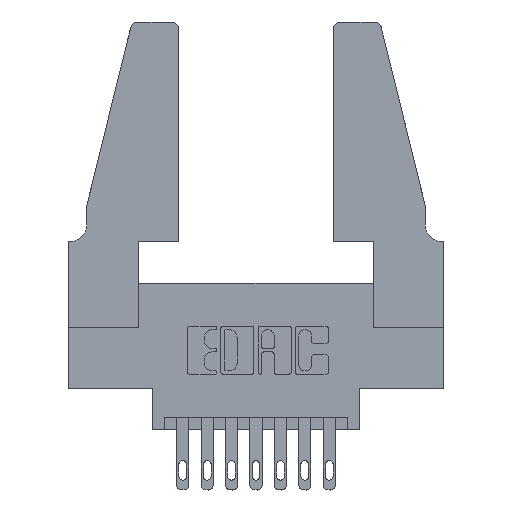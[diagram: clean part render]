
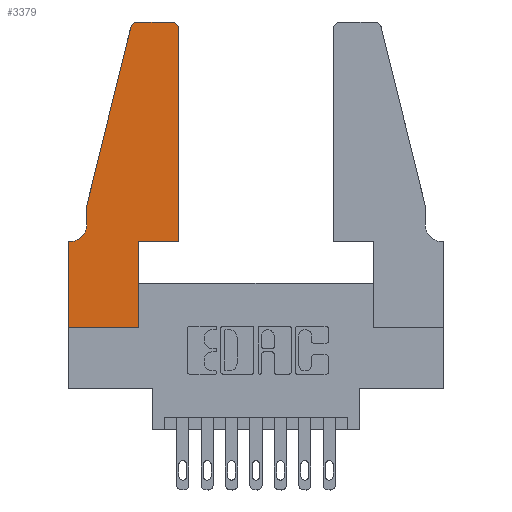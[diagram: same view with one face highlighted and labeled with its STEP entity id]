
A CAD part, top view. The second image highlights one B-rep face of the part: STEP entity #3379.
In plain terms, the highlighted planar face has unit normal (0, 0, 1).
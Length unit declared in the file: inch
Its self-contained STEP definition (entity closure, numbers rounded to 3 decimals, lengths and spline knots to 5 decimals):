
#151 = DIRECTION ( 'NONE',  ( 0., 1., 0. ) ) ;
#263 = DIRECTION ( 'NONE',  ( 0., -1., 0. ) ) ;
#394 = VECTOR ( 'NONE', #263, 39.37008 ) ;
#399 = CARTESIAN_POINT ( 'NONE',  ( 0.0055, 0.42, 0.37 ) ) ;
#408 = DIRECTION ( 'NONE',  ( 1., 0., 0. ) ) ;
#627 = VERTEX_POINT ( 'NONE', #6410 ) ;
#666 = ORIENTED_EDGE ( 'NONE', *, *, #2620, .T. ) ;
#720 = ORIENTED_EDGE ( 'NONE', *, *, #2877, .T. ) ;
#844 = LINE ( 'NONE', #12248, #8584 ) ;
#960 = VERTEX_POINT ( 'NONE', #8998 ) ;
#1277 = EDGE_CURVE ( 'NONE', #9759, #10800, #11972, .T. ) ;
#1378 = CIRCLE ( 'NONE', #9763, 0.03 ) ;
#1559 = DIRECTION ( 'NONE',  ( 0., 0., 1. ) ) ;
#1564 = VERTEX_POINT ( 'NONE', #7573 ) ;
#1573 = LINE ( 'NONE', #2717, #11346 ) ;
#2007 = EDGE_CURVE ( 'NONE', #4205, #9759, #9838, .T. ) ;
#2132 = CARTESIAN_POINT ( 'NONE',  ( 0.0755, 0.5, 0.37 ) ) ;
#2360 = DIRECTION ( 'NONE',  ( -1., 0., 0. ) ) ;
#2440 = CARTESIAN_POINT ( 'NONE',  ( 0.4505, 0.35, 0.37 ) ) ;
#2479 = EDGE_LOOP ( 'NONE', ( #9526, #11867, #720, #11897, #666, #7391, #10281, #10313, #12401, #6787, #3564, #7150 ) ) ;
#2620 = EDGE_CURVE ( 'NONE', #11312, #627, #8734, .T. ) ;
#2667 = EDGE_CURVE ( 'NONE', #7361, #6840, #6149, .T. ) ;
#2685 = CARTESIAN_POINT ( 'NONE',  ( 0.2865, 0.35, 0.37 ) ) ;
#2717 = CARTESIAN_POINT ( 'NONE',  ( 0., 0., 0.37 ) ) ;
#2877 = EDGE_CURVE ( 'NONE', #11779, #3362, #3349, .T. ) ;
#2882 = EDGE_CURVE ( 'NONE', #6840, #4205, #844, .T. ) ;
#3102 = DIRECTION ( 'NONE',  ( -0.239, -0.971, 0. ) ) ;
#3179 = CARTESIAN_POINT ( 'NONE',  ( 0.284, 1.22, 0.37 ) ) ;
#3225 = EDGE_CURVE ( 'NONE', #960, #1564, #1573, .T. ) ;
#3349 = LINE ( 'NONE', #2132, #10439 ) ;
#3362 = VERTEX_POINT ( 'NONE', #5424 ) ;
#3379 = ADVANCED_FACE ( 'NONE', ( #6712 ), #8198, .T. ) ;
#3395 = DIRECTION ( 'NONE',  ( 1., 0., 0. ) ) ;
#3564 = ORIENTED_EDGE ( 'NONE', *, *, #2882, .T. ) ;
#3666 = VECTOR ( 'NONE', #12202, 39.37008 ) ;
#3758 = LINE ( 'NONE', #6858, #8691 ) ;
#3938 = EDGE_CURVE ( 'NONE', #1564, #10353, #3758, .T. ) ;
#4205 = VERTEX_POINT ( 'NONE', #11463 ) ;
#4459 = DIRECTION ( 'NONE',  ( 1., 0., 0. ) ) ;
#4490 = EDGE_CURVE ( 'NONE', #10800, #11779, #1378, .T. ) ;
#4528 = AXIS2_PLACEMENT_3D ( 'NONE', #11253, #5376, #4459 ) ;
#4982 = CARTESIAN_POINT ( 'NONE',  ( 0.4505, 0.35, 0.37 ) ) ;
#5376 = DIRECTION ( 'NONE',  ( 0., 0., 1. ) ) ;
#5398 = AXIS2_PLACEMENT_3D ( 'NONE', #399, #10962, #2360 ) ;
#5424 = CARTESIAN_POINT ( 'NONE',  ( 0.0755, 0.5, 0.37 ) ) ;
#6149 = LINE ( 'NONE', #4982, #10115 ) ;
#6180 = LINE ( 'NONE', #8778, #394 ) ;
#6309 = DIRECTION ( 'NONE',  ( 1., 0., 0. ) ) ;
#6410 = CARTESIAN_POINT ( 'NONE',  ( 0.0055, 0.35, 0.37 ) ) ;
#6712 = FACE_OUTER_BOUND ( 'NONE', #2479, .T. ) ;
#6787 = ORIENTED_EDGE ( 'NONE', *, *, #2667, .T. ) ;
#6840 = VERTEX_POINT ( 'NONE', #2440 ) ;
#6858 = CARTESIAN_POINT ( 'NONE',  ( 0., 0., 0.37 ) ) ;
#7019 = EDGE_CURVE ( 'NONE', #10353, #7361, #9715, .T. ) ;
#7150 = ORIENTED_EDGE ( 'NONE', *, *, #2007, .T. ) ;
#7361 = VERTEX_POINT ( 'NONE', #9119 ) ;
#7391 = ORIENTED_EDGE ( 'NONE', *, *, #8482, .T. ) ;
#7534 = CARTESIAN_POINT ( 'NONE',  ( 0.284, 1.25, 0.37 ) ) ;
#7573 = CARTESIAN_POINT ( 'NONE',  ( 0., 0., 0.37 ) ) ;
#7779 = DIRECTION ( 'NONE',  ( 1., 0., 0. ) ) ;
#7996 = EDGE_CURVE ( 'NONE', #3362, #11312, #6180, .T. ) ;
#8040 = CARTESIAN_POINT ( 'NONE',  ( 0.0755, 0.42, 0.37 ) ) ;
#8079 = CARTESIAN_POINT ( 'NONE',  ( 0.2865, 0., 0.37 ) ) ;
#8115 = CARTESIAN_POINT ( 'NONE',  ( 0.25487, 1.22718, 0.37 ) ) ;
#8198 = PLANE ( 'NONE',  #4528 ) ;
#8295 = VECTOR ( 'NONE', #12144, 39.37008 ) ;
#8482 = EDGE_CURVE ( 'NONE', #627, #960, #12272, .T. ) ;
#8584 = VECTOR ( 'NONE', #151, 39.37008 ) ;
#8691 = VECTOR ( 'NONE', #408, 39.37008 ) ;
#8734 = CIRCLE ( 'NONE', #5398, 0.07 ) ;
#8778 = CARTESIAN_POINT ( 'NONE',  ( 0.0755, 0.5, 0.37 ) ) ;
#8795 = CARTESIAN_POINT ( 'NONE',  ( 0.4205, 1.25, 0.37 ) ) ;
#8998 = CARTESIAN_POINT ( 'NONE',  ( 0., 0.35, 0.37 ) ) ;
#9119 = CARTESIAN_POINT ( 'NONE',  ( 0.2865, 0.35, 0.37 ) ) ;
#9526 = ORIENTED_EDGE ( 'NONE', *, *, #1277, .T. ) ;
#9715 = LINE ( 'NONE', #2685, #11252 ) ;
#9759 = VERTEX_POINT ( 'NONE', #8795 ) ;
#9763 = AXIS2_PLACEMENT_3D ( 'NONE', #3179, #9781, #3395 ) ;
#9781 = DIRECTION ( 'NONE',  ( 0., 0., 1. ) ) ;
#9838 = CIRCLE ( 'NONE', #11766, 0.03 ) ;
#10115 = VECTOR ( 'NONE', #7779, 39.37008 ) ;
#10281 = ORIENTED_EDGE ( 'NONE', *, *, #3225, .T. ) ;
#10286 = CARTESIAN_POINT ( 'NONE',  ( 0.0755, 0.35, 0.37 ) ) ;
#10313 = ORIENTED_EDGE ( 'NONE', *, *, #3938, .T. ) ;
#10353 = VERTEX_POINT ( 'NONE', #8079 ) ;
#10439 = VECTOR ( 'NONE', #3102, 39.37008 ) ;
#10800 = VERTEX_POINT ( 'NONE', #7534 ) ;
#10962 = DIRECTION ( 'NONE',  ( 0., 0., -1. ) ) ;
#11252 = VECTOR ( 'NONE', #12403, 39.37008 ) ;
#11253 = CARTESIAN_POINT ( 'NONE',  ( 0., 0.35, 0.37 ) ) ;
#11312 = VERTEX_POINT ( 'NONE', #8040 ) ;
#11346 = VECTOR ( 'NONE', #12383, 39.37008 ) ;
#11463 = CARTESIAN_POINT ( 'NONE',  ( 0.4505, 1.22, 0.37 ) ) ;
#11766 = AXIS2_PLACEMENT_3D ( 'NONE', #12145, #1559, #6309 ) ;
#11779 = VERTEX_POINT ( 'NONE', #8115 ) ;
#11867 = ORIENTED_EDGE ( 'NONE', *, *, #4490, .T. ) ;
#11897 = ORIENTED_EDGE ( 'NONE', *, *, #7996, .T. ) ;
#11972 = LINE ( 'NONE', #12287, #3666 ) ;
#12144 = DIRECTION ( 'NONE',  ( -1., 0., 0. ) ) ;
#12145 = CARTESIAN_POINT ( 'NONE',  ( 0.4205, 1.22, 0.37 ) ) ;
#12202 = DIRECTION ( 'NONE',  ( -1., 0., 0. ) ) ;
#12248 = CARTESIAN_POINT ( 'NONE',  ( 0.4505, 0.35, 0.37 ) ) ;
#12272 = LINE ( 'NONE', #10286, #8295 ) ;
#12287 = CARTESIAN_POINT ( 'NONE',  ( 0.2605, 1.25, 0.37 ) ) ;
#12383 = DIRECTION ( 'NONE',  ( 0., -1., 0. ) ) ;
#12401 = ORIENTED_EDGE ( 'NONE', *, *, #7019, .T. ) ;
#12403 = DIRECTION ( 'NONE',  ( 0., 1., 0. ) ) ;
